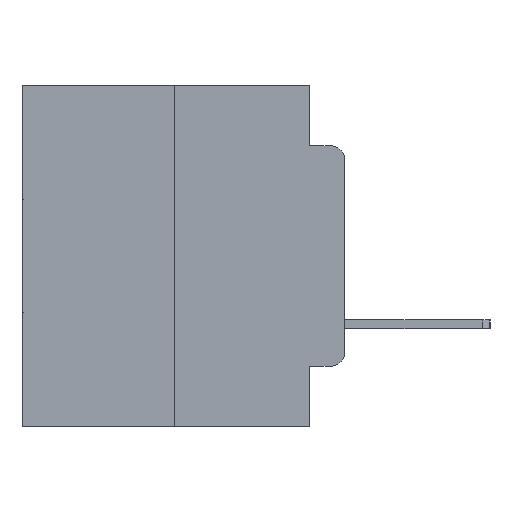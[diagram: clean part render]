
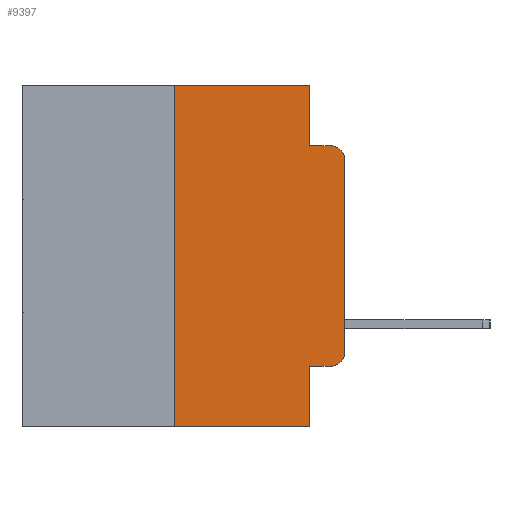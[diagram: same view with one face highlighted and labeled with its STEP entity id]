
A CAD part, left-side view. The second image highlights one B-rep face of the part: STEP entity #9397.
In plain terms, the highlighted planar face has unit normal (-1, 0, 0).
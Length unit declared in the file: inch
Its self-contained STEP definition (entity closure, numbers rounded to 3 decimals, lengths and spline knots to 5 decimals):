
#612 = ORIENTED_EDGE ( 'NONE', *, *, #4665, .F. ) ;
#660 = CARTESIAN_POINT ( 'NONE',  ( 0., 0.051, -0.5 ) ) ;
#666 = CARTESIAN_POINT ( 'NONE',  ( 0., 0.02, -0.4115 ) ) ;
#724 = AXIS2_PLACEMENT_3D ( 'NONE', #24576, #7474, #22565 ) ;
#786 = DIRECTION ( 'NONE',  ( 0., -1., 0. ) ) ;
#803 = VECTOR ( 'NONE', #10842, 39.37008 ) ;
#1053 = VERTEX_POINT ( 'NONE', #13064 ) ;
#1251 = VERTEX_POINT ( 'NONE', #22468 ) ;
#1268 = EDGE_CURVE ( 'NONE', #9095, #2765, #17041, .T. ) ;
#1750 = DIRECTION ( 'NONE',  ( 0., 0., -1. ) ) ;
#2028 = ORIENTED_EDGE ( 'NONE', *, *, #27010, .T. ) ;
#2765 = VERTEX_POINT ( 'NONE', #660 ) ;
#3209 = DIRECTION ( 'NONE',  ( -1., 0., 0. ) ) ;
#3288 = EDGE_LOOP ( 'NONE', ( #23821, #14600, #12195, #24823, #612, #18258, #2028, #10162, #11527, #22890 ) ) ;
#3767 = VECTOR ( 'NONE', #23374, 39.37008 ) ;
#4385 = VERTEX_POINT ( 'NONE', #666 ) ;
#4665 = EDGE_CURVE ( 'NONE', #17884, #1053, #7022, .T. ) ;
#4788 = CARTESIAN_POINT ( 'NONE',  ( 0., 0., -0.3915 ) ) ;
#5452 = DIRECTION ( 'NONE',  ( 0., 0., -1. ) ) ;
#5871 = AXIS2_PLACEMENT_3D ( 'NONE', #16521, #3209, #18618 ) ;
#5907 = EDGE_CURVE ( 'NONE', #19182, #6937, #12859, .T. ) ;
#5984 = VERTEX_POINT ( 'NONE', #27493 ) ;
#6062 = CARTESIAN_POINT ( 'NONE',  ( 0., 0.473, -0.5 ) ) ;
#6934 = VECTOR ( 'NONE', #14711, 39.37008 ) ;
#6937 = VERTEX_POINT ( 'NONE', #25145 ) ;
#7022 = LINE ( 'NONE', #11985, #23563 ) ;
#7276 = CARTESIAN_POINT ( 'NONE',  ( 0., 0.051, -0.4115 ) ) ;
#7330 = EDGE_CURVE ( 'NONE', #5984, #17884, #23381, .T. ) ;
#7401 = DIRECTION ( 'NONE',  ( 0., -1., 0. ) ) ;
#7474 = DIRECTION ( 'NONE',  ( 1., 0., 0. ) ) ;
#8233 = CARTESIAN_POINT ( 'NONE',  ( 0., 0.25, 0. ) ) ;
#9095 = VERTEX_POINT ( 'NONE', #22400 ) ;
#9397 = ADVANCED_FACE ( 'NONE', ( #19063 ), #26610, .F. ) ;
#9982 = CARTESIAN_POINT ( 'NONE',  ( 0., 0.051, 0. ) ) ;
#10162 = ORIENTED_EDGE ( 'NONE', *, *, #1268, .F. ) ;
#10218 = VECTOR ( 'NONE', #24483, 39.37008 ) ;
#10842 = DIRECTION ( 'NONE',  ( 0., 0., 1. ) ) ;
#10898 = EDGE_CURVE ( 'NONE', #9095, #4385, #22266, .T. ) ;
#10990 = EDGE_CURVE ( 'NONE', #6937, #1251, #13979, .T. ) ;
#11410 = VERTEX_POINT ( 'NONE', #24546 ) ;
#11527 = ORIENTED_EDGE ( 'NONE', *, *, #10898, .T. ) ;
#11866 = CARTESIAN_POINT ( 'NONE',  ( 0., 0.051, -0.0885 ) ) ;
#11985 = CARTESIAN_POINT ( 'NONE',  ( 0., 0.473, 0. ) ) ;
#12195 = ORIENTED_EDGE ( 'NONE', *, *, #28138, .F. ) ;
#12859 = LINE ( 'NONE', #18853, #6934 ) ;
#13064 = CARTESIAN_POINT ( 'NONE',  ( 0., 0.051, 0. ) ) ;
#13979 = CIRCLE ( 'NONE', #5871, 0.02 ) ;
#14194 = LINE ( 'NONE', #11866, #24749 ) ;
#14385 = EDGE_CURVE ( 'NONE', #4385, #19182, #19681, .T. ) ;
#14600 = ORIENTED_EDGE ( 'NONE', *, *, #10990, .T. ) ;
#14711 = DIRECTION ( 'NONE',  ( 0., 0., 1. ) ) ;
#15127 = DIRECTION ( 'NONE',  ( -1., 0., 0. ) ) ;
#16521 = CARTESIAN_POINT ( 'NONE',  ( 0., 0.02, -0.1085 ) ) ;
#17041 = LINE ( 'NONE', #18308, #27525 ) ;
#17884 = VERTEX_POINT ( 'NONE', #8233 ) ;
#18258 = ORIENTED_EDGE ( 'NONE', *, *, #7330, .F. ) ;
#18308 = CARTESIAN_POINT ( 'NONE',  ( 0., 0.051, 0. ) ) ;
#18618 = DIRECTION ( 'NONE',  ( 0., 0., -1. ) ) ;
#18853 = CARTESIAN_POINT ( 'NONE',  ( 0., 0., 0. ) ) ;
#19063 = FACE_OUTER_BOUND ( 'NONE', #3288, .T. ) ;
#19182 = VERTEX_POINT ( 'NONE', #4788 ) ;
#19681 = CIRCLE ( 'NONE', #20898, 0.02 ) ;
#19749 = DIRECTION ( 'NONE',  ( 0., 0., -1. ) ) ;
#20898 = AXIS2_PLACEMENT_3D ( 'NONE', #27692, #15127, #1750 ) ;
#22266 = LINE ( 'NONE', #7276, #10218 ) ;
#22400 = CARTESIAN_POINT ( 'NONE',  ( 0., 0.051, -0.4115 ) ) ;
#22468 = CARTESIAN_POINT ( 'NONE',  ( 0., 0.02, -0.0885 ) ) ;
#22565 = DIRECTION ( 'NONE',  ( 0., 0., -1. ) ) ;
#22890 = ORIENTED_EDGE ( 'NONE', *, *, #14385, .T. ) ;
#23374 = DIRECTION ( 'NONE',  ( 0., -1., 0. ) ) ;
#23381 = LINE ( 'NONE', #23629, #803 ) ;
#23563 = VECTOR ( 'NONE', #786, 39.37008 ) ;
#23629 = CARTESIAN_POINT ( 'NONE',  ( 0., 0.25, 0. ) ) ;
#23821 = ORIENTED_EDGE ( 'NONE', *, *, #5907, .T. ) ;
#24455 = VECTOR ( 'NONE', #5452, 39.37008 ) ;
#24483 = DIRECTION ( 'NONE',  ( 0., -1., 0. ) ) ;
#24546 = CARTESIAN_POINT ( 'NONE',  ( 0., 0.051, -0.0885 ) ) ;
#24576 = CARTESIAN_POINT ( 'NONE',  ( 0., 0.473, 0. ) ) ;
#24749 = VECTOR ( 'NONE', #7401, 39.37008 ) ;
#24823 = ORIENTED_EDGE ( 'NONE', *, *, #27445, .F. ) ;
#25134 = LINE ( 'NONE', #9982, #24455 ) ;
#25145 = CARTESIAN_POINT ( 'NONE',  ( 0., 0., -0.1085 ) ) ;
#26610 = PLANE ( 'NONE',  #724 ) ;
#26786 = LINE ( 'NONE', #6062, #3767 ) ;
#27010 = EDGE_CURVE ( 'NONE', #5984, #2765, #26786, .T. ) ;
#27445 = EDGE_CURVE ( 'NONE', #1053, #11410, #25134, .T. ) ;
#27493 = CARTESIAN_POINT ( 'NONE',  ( 0., 0.25, -0.5 ) ) ;
#27525 = VECTOR ( 'NONE', #19749, 39.37008 ) ;
#27692 = CARTESIAN_POINT ( 'NONE',  ( 0., 0.02, -0.3915 ) ) ;
#28138 = EDGE_CURVE ( 'NONE', #11410, #1251, #14194, .T. ) ;
